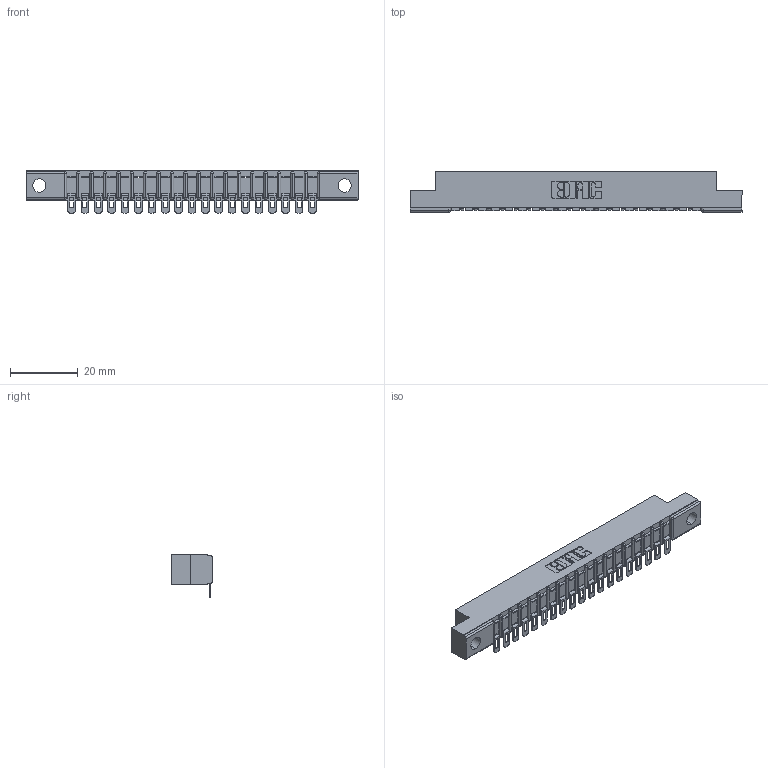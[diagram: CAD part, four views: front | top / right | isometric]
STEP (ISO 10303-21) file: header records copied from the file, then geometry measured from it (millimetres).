
FILE_DESCRIPTION (( 'STEP AP203' ), '1' );
FILE_NAME ('307-019-454-104.STEP', '2020-09-27T01:12:37', ( '' ), ( '' ), 'SwSTEP 2.0', 'SolidWorks 2020', '' );
FILE_SCHEMA (( 'CONFIG_CONTROL_DESIGN' ));
Length unit declared in the file: inch
Products named in the file (3): 307-019-454-104; 307-290-002_554; 307 Part_.156 Dia Mounting Holes
Assembly tree (20 placements, depth 2):
  307-019-454-104
    307 Part_.156 Dia Mounting Holes
    307-290-002_554  x19
Bounding box: 98.3 x 12.01 x 12.52 mm (x, y, z)
Volume: 6388.8 mm3; surface area: 11422.2 mm2
Topology: 20 solids, 20 shells, 1691 faces, 5166 edges, 3388 vertices
Faces by surface type: plane 958, cylinder 693, sphere 40
Entity records: 20507 total; most frequent: CARTESIAN_POINT 3460, ORIENTED_EDGE 3448, DIRECTION 3370, EDGE_CURVE 1724, VECTOR 1310, LINE 1310, VERTEX_POINT 1120, AXIS2_PLACEMENT_3D 1030
